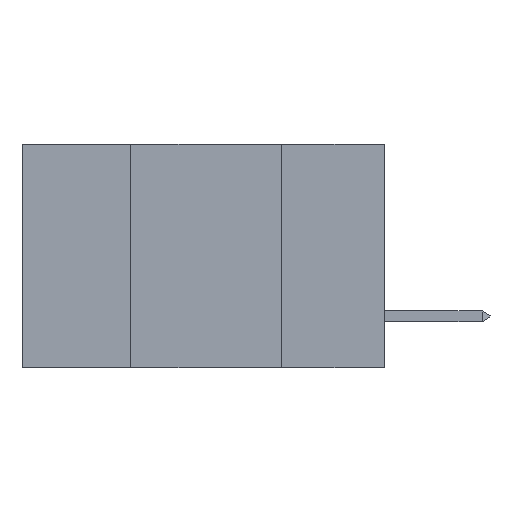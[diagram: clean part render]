
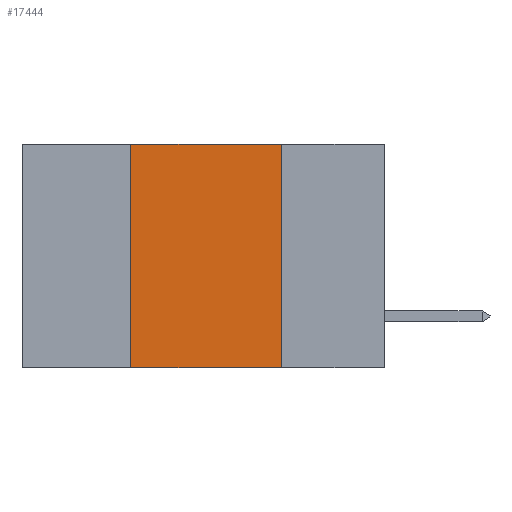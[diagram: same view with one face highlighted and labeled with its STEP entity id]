
A CAD part, left-side view. The second image highlights one B-rep face of the part: STEP entity #17444.
In plain terms, the highlighted planar face has unit normal (-1, 0, 0).
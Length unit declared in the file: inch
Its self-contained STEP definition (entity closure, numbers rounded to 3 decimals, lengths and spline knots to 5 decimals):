
#82 = VERTEX_POINT ( 'NONE', #3206 ) ;
#524 = EDGE_CURVE ( 'NONE', #14627, #11660, #6993, .T. ) ;
#1040 = DIRECTION ( 'NONE',  ( 0., 0., 1. ) ) ;
#1781 = DIRECTION ( 'NONE',  ( 0., 0., -1. ) ) ;
#3206 = CARTESIAN_POINT ( 'NONE',  ( 0., 0.42, -0.37 ) ) ;
#3351 = VECTOR ( 'NONE', #1781, 39.37008 ) ;
#3454 = FACE_OUTER_BOUND ( 'NONE', #8677, .T. ) ;
#3711 = ORIENTED_EDGE ( 'NONE', *, *, #10646, .F. ) ;
#3980 = VERTEX_POINT ( 'NONE', #10299 ) ;
#4192 = LINE ( 'NONE', #12308, #6694 ) ;
#4279 = DIRECTION ( 'NONE',  ( 0., -1., 0. ) ) ;
#5169 = LINE ( 'NONE', #11705, #13959 ) ;
#6095 = DIRECTION ( 'NONE',  ( 0., 0., -1. ) ) ;
#6185 = CARTESIAN_POINT ( 'NONE',  ( 0., 0.6, 0. ) ) ;
#6694 = VECTOR ( 'NONE', #4279, 39.37008 ) ;
#6983 = EDGE_CURVE ( 'NONE', #82, #11660, #5169, .T. ) ;
#6993 = LINE ( 'NONE', #16696, #3351 ) ;
#7240 = VECTOR ( 'NONE', #1040, 39.37008 ) ;
#7727 = ORIENTED_EDGE ( 'NONE', *, *, #11469, .F. ) ;
#8198 = CARTESIAN_POINT ( 'NONE',  ( 0., 0.42, 0. ) ) ;
#8292 = CARTESIAN_POINT ( 'NONE',  ( 0., 0.17, 0. ) ) ;
#8489 = AXIS2_PLACEMENT_3D ( 'NONE', #6185, #8833, #6095 ) ;
#8677 = EDGE_LOOP ( 'NONE', ( #11106, #7727, #3711, #9816 ) ) ;
#8833 = DIRECTION ( 'NONE',  ( 1., 0., 0. ) ) ;
#9231 = DIRECTION ( 'NONE',  ( 0., -1., 0. ) ) ;
#9816 = ORIENTED_EDGE ( 'NONE', *, *, #6983, .T. ) ;
#10299 = CARTESIAN_POINT ( 'NONE',  ( 0., 0.42, 0. ) ) ;
#10646 = EDGE_CURVE ( 'NONE', #82, #3980, #14645, .T. ) ;
#11106 = ORIENTED_EDGE ( 'NONE', *, *, #524, .F. ) ;
#11469 = EDGE_CURVE ( 'NONE', #3980, #14627, #4192, .T. ) ;
#11660 = VERTEX_POINT ( 'NONE', #12739 ) ;
#11705 = CARTESIAN_POINT ( 'NONE',  ( 0., 0.6, -0.37 ) ) ;
#12308 = CARTESIAN_POINT ( 'NONE',  ( 0., 0.6, 0. ) ) ;
#12739 = CARTESIAN_POINT ( 'NONE',  ( 0., 0.17, -0.37 ) ) ;
#13959 = VECTOR ( 'NONE', #9231, 39.37008 ) ;
#14309 = PLANE ( 'NONE',  #8489 ) ;
#14627 = VERTEX_POINT ( 'NONE', #8292 ) ;
#14645 = LINE ( 'NONE', #8198, #7240 ) ;
#16696 = CARTESIAN_POINT ( 'NONE',  ( 0., 0.17, 0. ) ) ;
#17444 = ADVANCED_FACE ( 'NONE', ( #3454 ), #14309, .F. ) ;
